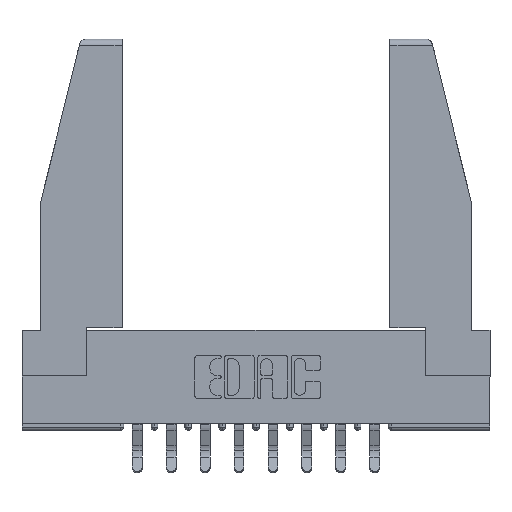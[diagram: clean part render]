
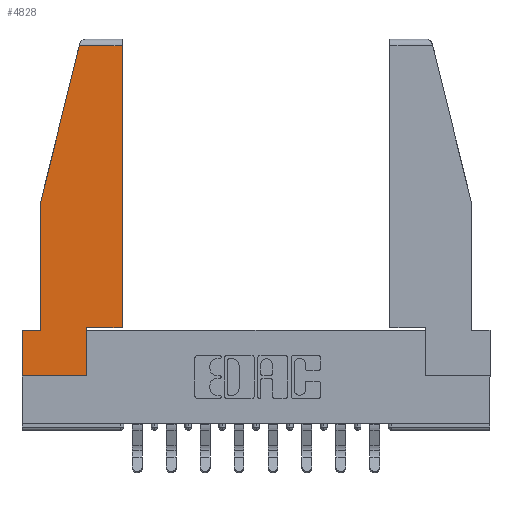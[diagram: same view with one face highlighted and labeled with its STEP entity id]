
A CAD part, top view. The second image highlights one B-rep face of the part: STEP entity #4828.
In plain terms, the highlighted planar face has unit normal (0, 0, 1).
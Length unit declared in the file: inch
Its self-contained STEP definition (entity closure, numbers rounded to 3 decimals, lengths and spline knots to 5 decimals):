
#106 = PLANE ( 'NONE',  #4301 ) ;
#541 = VECTOR ( 'NONE', #5888, 39.37008 ) ;
#872 = EDGE_CURVE ( 'NONE', #4347, #11668, #2806, .T. ) ;
#996 = VERTEX_POINT ( 'NONE', #13262 ) ;
#1094 = CARTESIAN_POINT ( 'NONE',  ( 0.297, 0., 0. ) ) ;
#1098 = CARTESIAN_POINT ( 'NONE',  ( 0., 1.52, 0. ) ) ;
#1577 = DIRECTION ( 'NONE',  ( 0., -1., 0. ) ) ;
#1609 = VERTEX_POINT ( 'NONE', #9705 ) ;
#1663 = CARTESIAN_POINT ( 'NONE',  ( 0.297, 0., 0. ) ) ;
#2162 = LINE ( 'NONE', #10860, #7379 ) ;
#2540 = DIRECTION ( 'NONE',  ( 1., 0., 0. ) ) ;
#2582 = VERTEX_POINT ( 'NONE', #9759 ) ;
#2587 = VERTEX_POINT ( 'NONE', #4914 ) ;
#2640 = ORIENTED_EDGE ( 'NONE', *, *, #3730, .T. ) ;
#2806 = LINE ( 'NONE', #1094, #541 ) ;
#3016 = DIRECTION ( 'NONE',  ( 1., 0., 0. ) ) ;
#3182 = VECTOR ( 'NONE', #12821, 39.37008 ) ;
#3201 = VERTEX_POINT ( 'NONE', #12771 ) ;
#3254 = VECTOR ( 'NONE', #1577, 39.37008 ) ;
#3602 = VECTOR ( 'NONE', #8357, 39.37008 ) ;
#3730 = EDGE_CURVE ( 'NONE', #4380, #2582, #2162, .T. ) ;
#4089 = CARTESIAN_POINT ( 'NONE',  ( 0., 0.21, 0. ) ) ;
#4117 = VECTOR ( 'NONE', #9701, 39.37008 ) ;
#4177 = ORIENTED_EDGE ( 'NONE', *, *, #7020, .T. ) ;
#4265 = CARTESIAN_POINT ( 'NONE',  ( 0., 0., 0. ) ) ;
#4301 = AXIS2_PLACEMENT_3D ( 'NONE', #8486, #10733, #2540 ) ;
#4347 = VERTEX_POINT ( 'NONE', #1663 ) ;
#4350 = CARTESIAN_POINT ( 'NONE',  ( 0.461, 0.223, 0. ) ) ;
#4380 = VERTEX_POINT ( 'NONE', #4350 ) ;
#4648 = VECTOR ( 'NONE', #3016, 39.37008 ) ;
#4654 = CARTESIAN_POINT ( 'NONE',  ( 0.086, 0.8, 0. ) ) ;
#4726 = ORIENTED_EDGE ( 'NONE', *, *, #8870, .T. ) ;
#4828 = ADVANCED_FACE ( 'NONE', ( #11656 ), #106, .T. ) ;
#4914 = CARTESIAN_POINT ( 'NONE',  ( 0., 0., 0. ) ) ;
#5044 = DIRECTION ( 'NONE',  ( 0., 1., 0. ) ) ;
#5306 = CARTESIAN_POINT ( 'NONE',  ( 0.297, 0.223, 0. ) ) ;
#5805 = EDGE_CURVE ( 'NONE', #11668, #4380, #9622, .T. ) ;
#5888 = DIRECTION ( 'NONE',  ( 0., 1., 0. ) ) ;
#6274 = VERTEX_POINT ( 'NONE', #6442 ) ;
#6442 = CARTESIAN_POINT ( 'NONE',  ( 0., 0.21, 0. ) ) ;
#6733 = LINE ( 'NONE', #4654, #3182 ) ;
#7020 = EDGE_CURVE ( 'NONE', #996, #1609, #6733, .T. ) ;
#7115 = EDGE_CURVE ( 'NONE', #3201, #996, #14910, .T. ) ;
#7379 = VECTOR ( 'NONE', #5044, 39.37008 ) ;
#7671 = CARTESIAN_POINT ( 'NONE',  ( 0., 0.21, 0. ) ) ;
#7901 = EDGE_CURVE ( 'NONE', #2587, #4347, #10459, .T. ) ;
#7983 = VECTOR ( 'NONE', #11181, 39.37008 ) ;
#8077 = EDGE_LOOP ( 'NONE', ( #2640, #8937, #9598, #4177, #4726, #14251, #13296, #11379, #10114 ) ) ;
#8357 = DIRECTION ( 'NONE',  ( -1., 0., 0. ) ) ;
#8486 = CARTESIAN_POINT ( 'NONE',  ( 0., 0., 0. ) ) ;
#8870 = EDGE_CURVE ( 'NONE', #1609, #6274, #14853, .T. ) ;
#8937 = ORIENTED_EDGE ( 'NONE', *, *, #12834, .T. ) ;
#9422 = VECTOR ( 'NONE', #13062, 39.37008 ) ;
#9598 = ORIENTED_EDGE ( 'NONE', *, *, #7115, .T. ) ;
#9622 = LINE ( 'NONE', #11838, #9422 ) ;
#9701 = DIRECTION ( 'NONE',  ( -0.239, -0.971, 0. ) ) ;
#9705 = CARTESIAN_POINT ( 'NONE',  ( 0.086, 0.21, 0. ) ) ;
#9759 = CARTESIAN_POINT ( 'NONE',  ( 0.461, 1.52, 0. ) ) ;
#10114 = ORIENTED_EDGE ( 'NONE', *, *, #5805, .T. ) ;
#10331 = CARTESIAN_POINT ( 'NONE',  ( 0.271, 1.55, 0. ) ) ;
#10459 = LINE ( 'NONE', #4265, #4648 ) ;
#10733 = DIRECTION ( 'NONE',  ( 0., 0., 1. ) ) ;
#10860 = CARTESIAN_POINT ( 'NONE',  ( 0.461, 0.223, 0. ) ) ;
#11181 = DIRECTION ( 'NONE',  ( -1., 0., 0. ) ) ;
#11379 = ORIENTED_EDGE ( 'NONE', *, *, #872, .T. ) ;
#11656 = FACE_OUTER_BOUND ( 'NONE', #8077, .T. ) ;
#11668 = VERTEX_POINT ( 'NONE', #5306 ) ;
#11750 = EDGE_CURVE ( 'NONE', #6274, #2587, #12553, .T. ) ;
#11838 = CARTESIAN_POINT ( 'NONE',  ( 0.297, 0.223, 0. ) ) ;
#12553 = LINE ( 'NONE', #7671, #3254 ) ;
#12771 = CARTESIAN_POINT ( 'NONE',  ( 0.2636, 1.52, 0. ) ) ;
#12821 = DIRECTION ( 'NONE',  ( 0., -1., 0. ) ) ;
#12834 = EDGE_CURVE ( 'NONE', #2582, #3201, #15344, .T. ) ;
#13062 = DIRECTION ( 'NONE',  ( 1., 0., 0. ) ) ;
#13262 = CARTESIAN_POINT ( 'NONE',  ( 0.086, 0.8, 0. ) ) ;
#13296 = ORIENTED_EDGE ( 'NONE', *, *, #7901, .T. ) ;
#14251 = ORIENTED_EDGE ( 'NONE', *, *, #11750, .T. ) ;
#14853 = LINE ( 'NONE', #4089, #7983 ) ;
#14910 = LINE ( 'NONE', #10331, #4117 ) ;
#15344 = LINE ( 'NONE', #1098, #3602 ) ;
